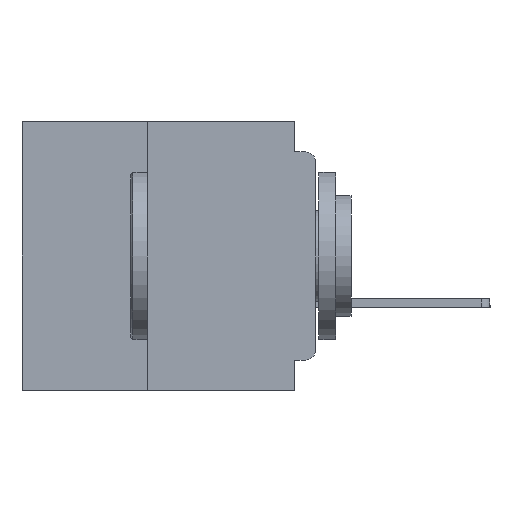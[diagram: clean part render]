
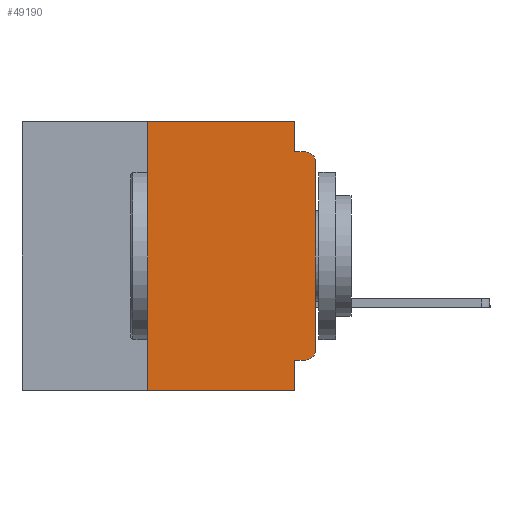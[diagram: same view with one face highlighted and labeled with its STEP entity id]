
A CAD part, left-side view. The second image highlights one B-rep face of the part: STEP entity #49190.
In plain terms, the highlighted planar face has unit normal (-1, 0, 0).
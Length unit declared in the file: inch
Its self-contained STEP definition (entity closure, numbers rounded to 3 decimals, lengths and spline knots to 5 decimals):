
#553 = CARTESIAN_POINT ( 'NONE',  ( 0., 0., -0.34 ) ) ;
#735 = LINE ( 'NONE', #34430, #42210 ) ;
#777 = LINE ( 'NONE', #23835, #43561 ) ;
#1196 = DIRECTION ( 'NONE',  ( 0., 1., 0. ) ) ;
#3633 = DIRECTION ( 'NONE',  ( 1., 0., 0. ) ) ;
#3781 = ORIENTED_EDGE ( 'NONE', *, *, #49610, .F. ) ;
#3789 = DIRECTION ( 'NONE',  ( 0., 0., -1. ) ) ;
#5770 = VECTOR ( 'NONE', #7249, 39.37008 ) ;
#5952 = EDGE_CURVE ( 'NONE', #51480, #26299, #40596, .T. ) ;
#6462 = DIRECTION ( 'NONE',  ( 0., 0., -1. ) ) ;
#7249 = DIRECTION ( 'NONE',  ( 0., 0., -1. ) ) ;
#7296 = CARTESIAN_POINT ( 'NONE',  ( 0., 0.031, 0. ) ) ;
#7449 = EDGE_CURVE ( 'NONE', #10966, #34511, #38431, .T. ) ;
#7595 = ORIENTED_EDGE ( 'NONE', *, *, #30422, .F. ) ;
#7836 = LINE ( 'NONE', #45122, #17514 ) ;
#8287 = ORIENTED_EDGE ( 'NONE', *, *, #27244, .F. ) ;
#8314 = VERTEX_POINT ( 'NONE', #40842 ) ;
#9270 = VECTOR ( 'NONE', #14491, 39.37008 ) ;
#9553 = EDGE_LOOP ( 'NONE', ( #46972, #37377, #53459, #3781, #8287, #24249, #28181, #22469, #7595, #13983 ) ) ;
#9566 = VECTOR ( 'NONE', #1196, 39.37008 ) ;
#9911 = DIRECTION ( 'NONE',  ( 0., -1., 0. ) ) ;
#10351 = VERTEX_POINT ( 'NONE', #38466 ) ;
#10595 = LINE ( 'NONE', #35184, #53349 ) ;
#10966 = VERTEX_POINT ( 'NONE', #42626 ) ;
#11243 = VERTEX_POINT ( 'NONE', #52879 ) ;
#13745 = VERTEX_POINT ( 'NONE', #48841 ) ;
#13983 = ORIENTED_EDGE ( 'NONE', *, *, #5952, .T. ) ;
#14469 = CARTESIAN_POINT ( 'NONE',  ( 0., 0.015, -0.06 ) ) ;
#14491 = DIRECTION ( 'NONE',  ( 0., 0., 1. ) ) ;
#16768 = LINE ( 'NONE', #52509, #5770 ) ;
#17514 = VECTOR ( 'NONE', #24444, 39.37008 ) ;
#17913 = EDGE_CURVE ( 'NONE', #53399, #8314, #19667, .T. ) ;
#18631 = DIRECTION ( 'NONE',  ( 0., 0., -1. ) ) ;
#19493 = EDGE_CURVE ( 'NONE', #53399, #13745, #7836, .T. ) ;
#19667 = LINE ( 'NONE', #34690, #43018 ) ;
#21093 = EDGE_CURVE ( 'NONE', #10351, #34511, #735, .T. ) ;
#21774 = CARTESIAN_POINT ( 'NONE',  ( 0., 0.25, -0.4 ) ) ;
#22469 = ORIENTED_EDGE ( 'NONE', *, *, #29505, .F. ) ;
#22974 = FACE_OUTER_BOUND ( 'NONE', #9553, .T. ) ;
#23266 = CARTESIAN_POINT ( 'NONE',  ( 0., 0.015, -0.045 ) ) ;
#23275 = VERTEX_POINT ( 'NONE', #7296 ) ;
#23835 = CARTESIAN_POINT ( 'NONE',  ( 0., 0.437, 0. ) ) ;
#24249 = ORIENTED_EDGE ( 'NONE', *, *, #19493, .F. ) ;
#24444 = DIRECTION ( 'NONE',  ( 0., 0., 1. ) ) ;
#24545 = AXIS2_PLACEMENT_3D ( 'NONE', #14469, #43485, #18631 ) ;
#26299 = VERTEX_POINT ( 'NONE', #553 ) ;
#27244 = EDGE_CURVE ( 'NONE', #13745, #23275, #777, .T. ) ;
#28181 = ORIENTED_EDGE ( 'NONE', *, *, #17913, .T. ) ;
#28545 = DIRECTION ( 'NONE',  ( -1., 0., 0. ) ) ;
#29505 = EDGE_CURVE ( 'NONE', #11243, #8314, #16768, .T. ) ;
#30422 = EDGE_CURVE ( 'NONE', #51480, #11243, #48458, .T. ) ;
#31269 = LINE ( 'NONE', #43508, #9270 ) ;
#32546 = DIRECTION ( 'NONE',  ( 0., 0., -1. ) ) ;
#34430 = CARTESIAN_POINT ( 'NONE',  ( 0., 0., -0.045 ) ) ;
#34511 = VERTEX_POINT ( 'NONE', #23266 ) ;
#34622 = DIRECTION ( 'NONE',  ( 0., -1., 0. ) ) ;
#34690 = CARTESIAN_POINT ( 'NONE',  ( 0., 0.437, -0.4 ) ) ;
#35184 = CARTESIAN_POINT ( 'NONE',  ( 0., 0.031, 0. ) ) ;
#36515 = CARTESIAN_POINT ( 'NONE',  ( 0., 0.437, 0. ) ) ;
#37377 = ORIENTED_EDGE ( 'NONE', *, *, #7449, .T. ) ;
#38431 = CIRCLE ( 'NONE', #24545, 0.015 ) ;
#38466 = CARTESIAN_POINT ( 'NONE',  ( 0., 0.031, -0.045 ) ) ;
#40596 = CIRCLE ( 'NONE', #52924, 0.015 ) ;
#40842 = CARTESIAN_POINT ( 'NONE',  ( 0., 0.031, -0.4 ) ) ;
#41170 = CARTESIAN_POINT ( 'NONE',  ( 0., 0.015, -0.355 ) ) ;
#42210 = VECTOR ( 'NONE', #34622, 39.37008 ) ;
#42626 = CARTESIAN_POINT ( 'NONE',  ( 0., 0., -0.06 ) ) ;
#43018 = VECTOR ( 'NONE', #9911, 39.37008 ) ;
#43485 = DIRECTION ( 'NONE',  ( -1., 0., 0. ) ) ;
#43508 = CARTESIAN_POINT ( 'NONE',  ( 0., 0., 0. ) ) ;
#43561 = VECTOR ( 'NONE', #48649, 39.37008 ) ;
#45122 = CARTESIAN_POINT ( 'NONE',  ( 0., 0.25, -0.4 ) ) ;
#46667 = CARTESIAN_POINT ( 'NONE',  ( 0., 0., -0.355 ) ) ;
#46972 = ORIENTED_EDGE ( 'NONE', *, *, #50727, .T. ) ;
#48458 = LINE ( 'NONE', #46667, #9566 ) ;
#48649 = DIRECTION ( 'NONE',  ( 0., -1., 0. ) ) ;
#48841 = CARTESIAN_POINT ( 'NONE',  ( 0., 0.25, 0. ) ) ;
#49190 = ADVANCED_FACE ( 'NONE', ( #22974 ), #53203, .F. ) ;
#49610 = EDGE_CURVE ( 'NONE', #23275, #10351, #10595, .T. ) ;
#50727 = EDGE_CURVE ( 'NONE', #26299, #10966, #31269, .T. ) ;
#51480 = VERTEX_POINT ( 'NONE', #41170 ) ;
#52509 = CARTESIAN_POINT ( 'NONE',  ( 0., 0.031, -0.4 ) ) ;
#52879 = CARTESIAN_POINT ( 'NONE',  ( 0., 0.031, -0.355 ) ) ;
#52924 = AXIS2_PLACEMENT_3D ( 'NONE', #53358, #28545, #3789 ) ;
#53203 = PLANE ( 'NONE',  #53436 ) ;
#53349 = VECTOR ( 'NONE', #6462, 39.37008 ) ;
#53358 = CARTESIAN_POINT ( 'NONE',  ( 0., 0.015, -0.34 ) ) ;
#53399 = VERTEX_POINT ( 'NONE', #21774 ) ;
#53436 = AXIS2_PLACEMENT_3D ( 'NONE', #36515, #3633, #32546 ) ;
#53459 = ORIENTED_EDGE ( 'NONE', *, *, #21093, .F. ) ;
